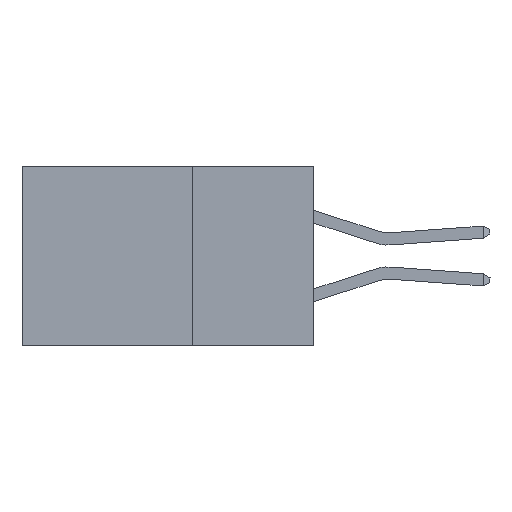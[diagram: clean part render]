
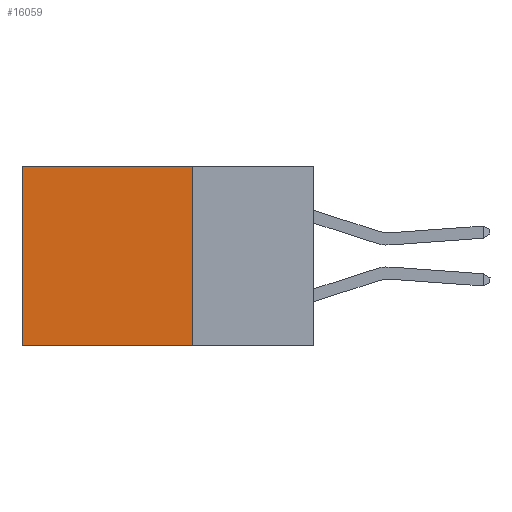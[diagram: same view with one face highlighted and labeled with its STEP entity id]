
A CAD part, left-side view. The second image highlights one B-rep face of the part: STEP entity #16059.
In plain terms, the highlighted planar face has unit normal (-1, 0, 0).
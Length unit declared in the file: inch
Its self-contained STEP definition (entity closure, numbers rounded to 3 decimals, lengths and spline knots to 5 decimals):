
#454 = ORIENTED_EDGE ( 'NONE', *, *, #12714, .F. ) ;
#811 = VERTEX_POINT ( 'NONE', #10443 ) ;
#1642 = EDGE_LOOP ( 'NONE', ( #13095, #454, #4078, #10748 ) ) ;
#2612 = DIRECTION ( 'NONE',  ( 1., 0., 0. ) ) ;
#3088 = CARTESIAN_POINT ( 'NONE',  ( 0.2875, 0.6, 0. ) ) ;
#3468 = LINE ( 'NONE', #8730, #8082 ) ;
#3527 = DIRECTION ( 'NONE',  ( 0., 0., -1. ) ) ;
#3956 = DIRECTION ( 'NONE',  ( 0., 1., 0. ) ) ;
#3979 = CARTESIAN_POINT ( 'NONE',  ( 0.2875, 0.25, -0.37 ) ) ;
#4078 = ORIENTED_EDGE ( 'NONE', *, *, #20123, .F. ) ;
#5209 = LINE ( 'NONE', #13841, #22515 ) ;
#5241 = EDGE_CURVE ( 'NONE', #15573, #14401, #5209, .T. ) ;
#8082 = VECTOR ( 'NONE', #3527, 39.37008 ) ;
#8730 = CARTESIAN_POINT ( 'NONE',  ( 0.2875, 0.25, 0. ) ) ;
#9899 = AXIS2_PLACEMENT_3D ( 'NONE', #16392, #2612, #14735 ) ;
#10420 = DIRECTION ( 'NONE',  ( 0., 0., -1. ) ) ;
#10443 = CARTESIAN_POINT ( 'NONE',  ( 0.2875, 0.25, 0. ) ) ;
#10748 = ORIENTED_EDGE ( 'NONE', *, *, #10839, .T. ) ;
#10839 = EDGE_CURVE ( 'NONE', #811, #15573, #12236, .T. ) ;
#12236 = LINE ( 'NONE', #21226, #15729 ) ;
#12714 = EDGE_CURVE ( 'NONE', #13027, #14401, #22161, .T. ) ;
#13021 = PLANE ( 'NONE',  #9899 ) ;
#13027 = VERTEX_POINT ( 'NONE', #18769 ) ;
#13095 = ORIENTED_EDGE ( 'NONE', *, *, #5241, .T. ) ;
#13507 = VECTOR ( 'NONE', #14338, 39.37008 ) ;
#13841 = CARTESIAN_POINT ( 'NONE',  ( 0.2875, 0.6, 0. ) ) ;
#14338 = DIRECTION ( 'NONE',  ( 0., 1., 0. ) ) ;
#14401 = VERTEX_POINT ( 'NONE', #19295 ) ;
#14735 = DIRECTION ( 'NONE',  ( 0., 0., -1. ) ) ;
#15573 = VERTEX_POINT ( 'NONE', #3088 ) ;
#15729 = VECTOR ( 'NONE', #3956, 39.37008 ) ;
#16059 = ADVANCED_FACE ( 'NONE', ( #21301 ), #13021, .F. ) ;
#16392 = CARTESIAN_POINT ( 'NONE',  ( 0.2875, 0.25, 0. ) ) ;
#18769 = CARTESIAN_POINT ( 'NONE',  ( 0.2875, 0.25, -0.37 ) ) ;
#19295 = CARTESIAN_POINT ( 'NONE',  ( 0.2875, 0.6, -0.37 ) ) ;
#20123 = EDGE_CURVE ( 'NONE', #811, #13027, #3468, .T. ) ;
#21226 = CARTESIAN_POINT ( 'NONE',  ( 0.2875, 0.25, 0. ) ) ;
#21301 = FACE_OUTER_BOUND ( 'NONE', #1642, .T. ) ;
#22161 = LINE ( 'NONE', #3979, #13507 ) ;
#22515 = VECTOR ( 'NONE', #10420, 39.37008 ) ;
